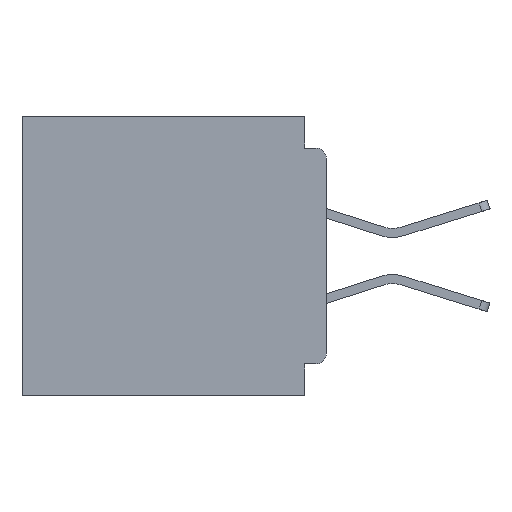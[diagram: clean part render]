
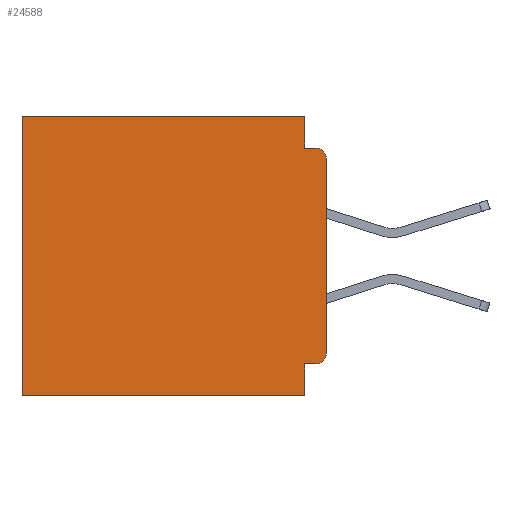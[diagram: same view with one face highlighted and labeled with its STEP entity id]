
A CAD part, left-side view. The second image highlights one B-rep face of the part: STEP entity #24588.
In plain terms, the highlighted planar face has unit normal (-1, 0, 0).
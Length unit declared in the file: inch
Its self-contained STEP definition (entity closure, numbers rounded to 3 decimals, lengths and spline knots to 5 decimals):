
#81 = CARTESIAN_POINT ( 'NONE',  ( 0.3, 0., -0.4 ) ) ;
#1750 = EDGE_CURVE ( 'NONE', #6832, #19817, #25462, .T. ) ;
#2132 = DIRECTION ( 'NONE',  ( 0., 0., -1. ) ) ;
#2263 = DIRECTION ( 'NONE',  ( 0., 0., -1. ) ) ;
#3234 = EDGE_CURVE ( 'NONE', #30416, #37665, #4119, .T. ) ;
#3610 = ORIENTED_EDGE ( 'NONE', *, *, #51981, .F. ) ;
#4119 = CIRCLE ( 'NONE', #50953, 0.015 ) ;
#4970 = ORIENTED_EDGE ( 'NONE', *, *, #6171, .F. ) ;
#6171 = EDGE_CURVE ( 'NONE', #16723, #28203, #54034, .T. ) ;
#6671 = CARTESIAN_POINT ( 'NONE',  ( 0.3, 0., -0.4 ) ) ;
#6832 = VERTEX_POINT ( 'NONE', #42479 ) ;
#9048 = CARTESIAN_POINT ( 'NONE',  ( 0.3, 0.437, -0.4 ) ) ;
#9576 = CARTESIAN_POINT ( 'NONE',  ( 0.3, 0., -0.06 ) ) ;
#10291 = VERTEX_POINT ( 'NONE', #18774 ) ;
#10498 = CARTESIAN_POINT ( 'NONE',  ( 0.3, 0.031, -0.045 ) ) ;
#10515 = CARTESIAN_POINT ( 'NONE',  ( 0.3, 0.015, -0.06 ) ) ;
#10908 = VECTOR ( 'NONE', #43793, 39.37008 ) ;
#11514 = VERTEX_POINT ( 'NONE', #32499 ) ;
#13150 = VECTOR ( 'NONE', #39899, 39.37008 ) ;
#13743 = ORIENTED_EDGE ( 'NONE', *, *, #3234, .T. ) ;
#14491 = ORIENTED_EDGE ( 'NONE', *, *, #55232, .T. ) ;
#15702 = CARTESIAN_POINT ( 'NONE',  ( 0.3, 0., 0. ) ) ;
#15897 = LINE ( 'NONE', #24336, #51539 ) ;
#16723 = VERTEX_POINT ( 'NONE', #36357 ) ;
#18229 = ORIENTED_EDGE ( 'NONE', *, *, #27882, .F. ) ;
#18774 = CARTESIAN_POINT ( 'NONE',  ( 0.3, 0., -0.34 ) ) ;
#19072 = DIRECTION ( 'NONE',  ( -1., 0., 0. ) ) ;
#19570 = ORIENTED_EDGE ( 'NONE', *, *, #51442, .F. ) ;
#19680 = DIRECTION ( 'NONE',  ( 0., 1., 0. ) ) ;
#19692 = DIRECTION ( 'NONE',  ( -1., 0., 0. ) ) ;
#19817 = VERTEX_POINT ( 'NONE', #31059 ) ;
#21727 = ORIENTED_EDGE ( 'NONE', *, *, #39569, .F. ) ;
#24336 = CARTESIAN_POINT ( 'NONE',  ( 0.3, 0., -0.355 ) ) ;
#24588 = ADVANCED_FACE ( 'NONE', ( #31933 ), #57927, .F. ) ;
#24628 = EDGE_LOOP ( 'NONE', ( #21727, #13743, #19570, #33421, #50140, #14491, #4970, #18229, #3610, #37210 ) ) ;
#25462 = LINE ( 'NONE', #15702, #13150 ) ;
#26224 = CIRCLE ( 'NONE', #27097, 0.015 ) ;
#26498 = DIRECTION ( 'NONE',  ( 0., 0., -1. ) ) ;
#27004 = CARTESIAN_POINT ( 'NONE',  ( 0.3, 0.031, 0. ) ) ;
#27097 = AXIS2_PLACEMENT_3D ( 'NONE', #46920, #19072, #51594 ) ;
#27882 = EDGE_CURVE ( 'NONE', #11514, #16723, #54022, .T. ) ;
#28036 = DIRECTION ( 'NONE',  ( 0., 0., -1. ) ) ;
#28126 = AXIS2_PLACEMENT_3D ( 'NONE', #6671, #30097, #2132 ) ;
#28203 = VERTEX_POINT ( 'NONE', #9048 ) ;
#28966 = CARTESIAN_POINT ( 'NONE',  ( 0.3, 0.015, -0.045 ) ) ;
#30097 = DIRECTION ( 'NONE',  ( 1., 0., 0. ) ) ;
#30416 = VERTEX_POINT ( 'NONE', #9576 ) ;
#30556 = VECTOR ( 'NONE', #50179, 39.37008 ) ;
#30757 = VECTOR ( 'NONE', #2263, 39.37008 ) ;
#31059 = CARTESIAN_POINT ( 'NONE',  ( 0.3, 0.437, 0. ) ) ;
#31520 = LINE ( 'NONE', #47743, #54774 ) ;
#31933 = FACE_OUTER_BOUND ( 'NONE', #24628, .T. ) ;
#32499 = CARTESIAN_POINT ( 'NONE',  ( 0.3, 0.031, -0.355 ) ) ;
#33421 = ORIENTED_EDGE ( 'NONE', *, *, #36747, .F. ) ;
#34401 = CARTESIAN_POINT ( 'NONE',  ( 0.3, 0., -0.045 ) ) ;
#36069 = DIRECTION ( 'NONE',  ( 0., 1., 0. ) ) ;
#36357 = CARTESIAN_POINT ( 'NONE',  ( 0.3, 0.031, -0.4 ) ) ;
#36747 = EDGE_CURVE ( 'NONE', #6832, #50596, #56725, .T. ) ;
#37210 = ORIENTED_EDGE ( 'NONE', *, *, #49986, .T. ) ;
#37665 = VERTEX_POINT ( 'NONE', #28966 ) ;
#38628 = DIRECTION ( 'NONE',  ( 0., 0., -1. ) ) ;
#39569 = EDGE_CURVE ( 'NONE', #30416, #10291, #50245, .T. ) ;
#39899 = DIRECTION ( 'NONE',  ( 0., 1., 0. ) ) ;
#40272 = VERTEX_POINT ( 'NONE', #42472 ) ;
#40750 = CARTESIAN_POINT ( 'NONE',  ( 0.3, 0., -0.4 ) ) ;
#42472 = CARTESIAN_POINT ( 'NONE',  ( 0.3, 0.015, -0.355 ) ) ;
#42479 = CARTESIAN_POINT ( 'NONE',  ( 0.3, 0.031, 0. ) ) ;
#43793 = DIRECTION ( 'NONE',  ( 0., -1., 0. ) ) ;
#46920 = CARTESIAN_POINT ( 'NONE',  ( 0.3, 0.015, -0.34 ) ) ;
#47317 = VECTOR ( 'NONE', #28036, 39.37008 ) ;
#47743 = CARTESIAN_POINT ( 'NONE',  ( 0.3, 0.437, -0.4 ) ) ;
#47974 = LINE ( 'NONE', #34401, #10908 ) ;
#49986 = EDGE_CURVE ( 'NONE', #40272, #10291, #26224, .T. ) ;
#50140 = ORIENTED_EDGE ( 'NONE', *, *, #1750, .T. ) ;
#50179 = DIRECTION ( 'NONE',  ( 0., 0., -1. ) ) ;
#50245 = LINE ( 'NONE', #81, #47317 ) ;
#50596 = VERTEX_POINT ( 'NONE', #10498 ) ;
#50953 = AXIS2_PLACEMENT_3D ( 'NONE', #10515, #19692, #26498 ) ;
#51442 = EDGE_CURVE ( 'NONE', #50596, #37665, #47974, .T. ) ;
#51539 = VECTOR ( 'NONE', #19680, 39.37008 ) ;
#51594 = DIRECTION ( 'NONE',  ( 0., 0., -1. ) ) ;
#51981 = EDGE_CURVE ( 'NONE', #40272, #11514, #15897, .T. ) ;
#52558 = VECTOR ( 'NONE', #36069, 39.37008 ) ;
#54022 = LINE ( 'NONE', #58052, #30757 ) ;
#54034 = LINE ( 'NONE', #40750, #52558 ) ;
#54774 = VECTOR ( 'NONE', #38628, 39.37008 ) ;
#55232 = EDGE_CURVE ( 'NONE', #19817, #28203, #31520, .T. ) ;
#56725 = LINE ( 'NONE', #27004, #30556 ) ;
#57927 = PLANE ( 'NONE',  #28126 ) ;
#58052 = CARTESIAN_POINT ( 'NONE',  ( 0.3, 0.031, -0.4 ) ) ;
